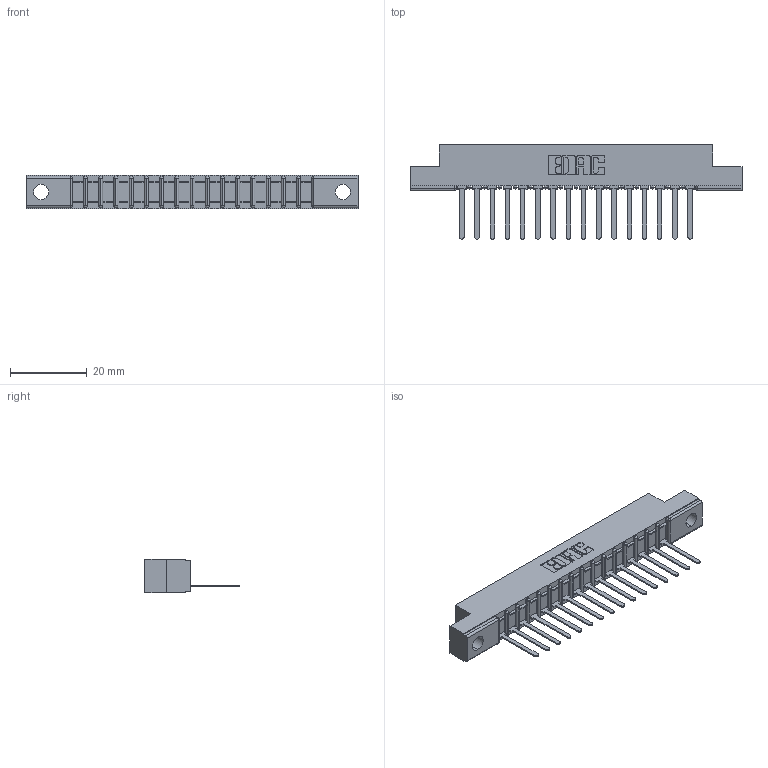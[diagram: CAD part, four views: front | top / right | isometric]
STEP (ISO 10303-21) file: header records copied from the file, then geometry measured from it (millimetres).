
FILE_DESCRIPTION (( 'STEP AP203' ), '1' );
FILE_NAME ('307-016-441-104.STEP', '2020-09-25T19:55:51', ( '' ), ( '' ), 'SwSTEP 2.0', 'SolidWorks 2020', '' );
FILE_SCHEMA (( 'CONFIG_CONTROL_DESIGN' ));
Length unit declared in the file: inch
Products named in the file (3): 307 Part_.156 Dia Mounting Holes; 307-016-441-104; 307-290-002_541
Assembly tree (17 placements, depth 2):
  307-016-441-104
    307 Part_.156 Dia Mounting Holes
    307-290-002_541  x16
Bounding box: 86.41 x 24.59 x 8.71 mm (x, y, z)
Volume: 5640.7 mm3; surface area: 10089.4 mm2
Topology: 17 solids, 17 shells, 1333 faces, 4071 edges, 2666 vertices
Faces by surface type: plane 804, cylinder 495, sphere 34
Entity records: 18058 total; most frequent: CARTESIAN_POINT 3046, ORIENTED_EDGE 3034, DIRECTION 2963, EDGE_CURVE 1517, VECTOR 1157, LINE 1157, VERTEX_POINT 986, AXIS2_PLACEMENT_3D 903
